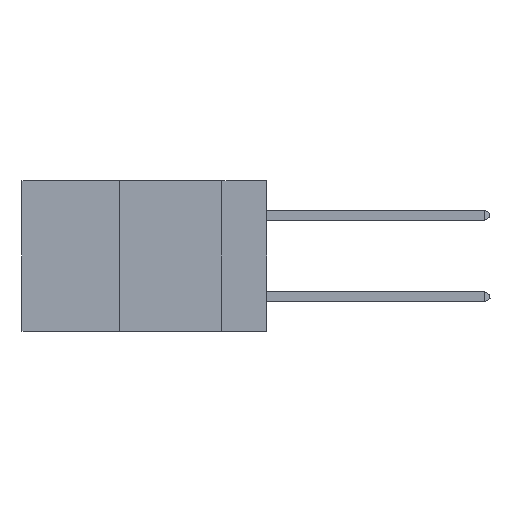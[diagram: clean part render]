
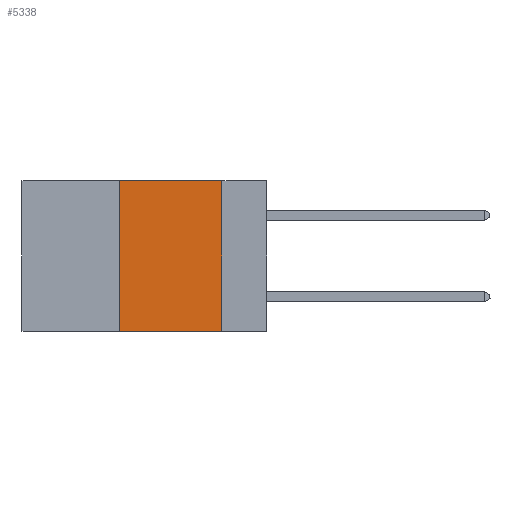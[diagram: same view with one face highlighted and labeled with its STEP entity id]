
A CAD part, left-side view. The second image highlights one B-rep face of the part: STEP entity #5338.
In plain terms, the highlighted planar face has unit normal (-1, 0, 0).
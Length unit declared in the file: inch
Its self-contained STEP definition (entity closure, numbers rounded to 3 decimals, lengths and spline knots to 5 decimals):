
#351 = VERTEX_POINT ( 'NONE', #6044 ) ;
#893 = ORIENTED_EDGE ( 'NONE', *, *, #1578, .T. ) ;
#977 = FACE_OUTER_BOUND ( 'NONE', #2028, .T. ) ;
#1091 = ORIENTED_EDGE ( 'NONE', *, *, #5289, .F. ) ;
#1187 = ORIENTED_EDGE ( 'NONE', *, *, #8458, .F. ) ;
#1238 = ORIENTED_EDGE ( 'NONE', *, *, #5328, .F. ) ;
#1578 = EDGE_CURVE ( 'NONE', #3052, #351, #4424, .T. ) ;
#1660 = VECTOR ( 'NONE', #2849, 39.37008 ) ;
#1754 = DIRECTION ( 'NONE',  ( 1., 0., 0. ) ) ;
#2028 = EDGE_LOOP ( 'NONE', ( #1091, #1187, #1238, #893 ) ) ;
#2316 = VECTOR ( 'NONE', #8988, 39.37008 ) ;
#2562 = PLANE ( 'NONE',  #2701 ) ;
#2631 = CARTESIAN_POINT ( 'NONE',  ( 0., 0.6, 0. ) ) ;
#2700 = CARTESIAN_POINT ( 'NONE',  ( 0., 0.6, -0.37 ) ) ;
#2701 = AXIS2_PLACEMENT_3D ( 'NONE', #2631, #1754, #5812 ) ;
#2743 = CARTESIAN_POINT ( 'NONE',  ( 0., 0.11, 0. ) ) ;
#2849 = DIRECTION ( 'NONE',  ( 0., -1., 0. ) ) ;
#3052 = VERTEX_POINT ( 'NONE', #9320 ) ;
#3411 = DIRECTION ( 'NONE',  ( 0., 0., 1. ) ) ;
#3449 = CARTESIAN_POINT ( 'NONE',  ( 0., 0.36, 0. ) ) ;
#4030 = LINE ( 'NONE', #8417, #1660 ) ;
#4424 = LINE ( 'NONE', #2700, #2316 ) ;
#4623 = DIRECTION ( 'NONE',  ( 0., 0., -1. ) ) ;
#4886 = CARTESIAN_POINT ( 'NONE',  ( 0., 0.36, 0. ) ) ;
#5289 = EDGE_CURVE ( 'NONE', #5602, #351, #5833, .T. ) ;
#5328 = EDGE_CURVE ( 'NONE', #3052, #8422, #8556, .T. ) ;
#5338 = ADVANCED_FACE ( 'NONE', ( #977 ), #2562, .F. ) ;
#5602 = VERTEX_POINT ( 'NONE', #2743 ) ;
#5812 = DIRECTION ( 'NONE',  ( 0., 0., -1. ) ) ;
#5833 = LINE ( 'NONE', #8625, #8567 ) ;
#6044 = CARTESIAN_POINT ( 'NONE',  ( 0., 0.11, -0.37 ) ) ;
#6443 = VECTOR ( 'NONE', #3411, 39.37008 ) ;
#8417 = CARTESIAN_POINT ( 'NONE',  ( 0., 0.6, 0. ) ) ;
#8422 = VERTEX_POINT ( 'NONE', #3449 ) ;
#8458 = EDGE_CURVE ( 'NONE', #8422, #5602, #4030, .T. ) ;
#8556 = LINE ( 'NONE', #4886, #6443 ) ;
#8567 = VECTOR ( 'NONE', #4623, 39.37008 ) ;
#8625 = CARTESIAN_POINT ( 'NONE',  ( 0., 0.11, 0. ) ) ;
#8988 = DIRECTION ( 'NONE',  ( 0., -1., 0. ) ) ;
#9320 = CARTESIAN_POINT ( 'NONE',  ( 0., 0.36, -0.37 ) ) ;
